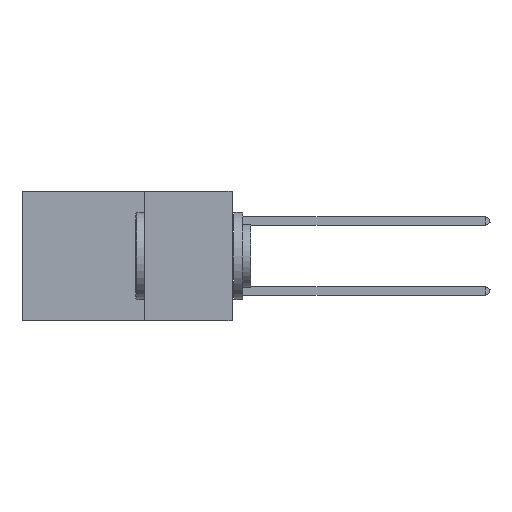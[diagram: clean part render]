
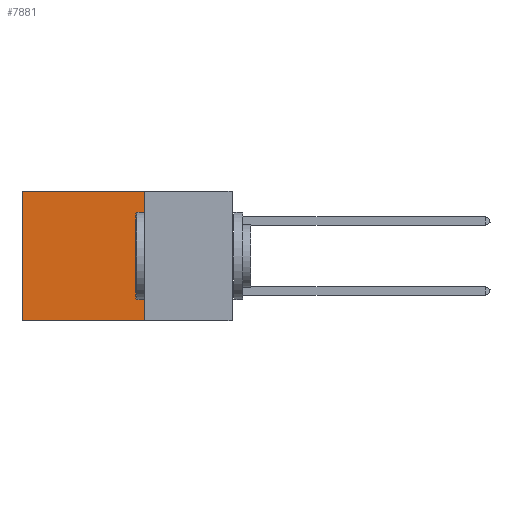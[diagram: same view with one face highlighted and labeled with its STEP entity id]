
A CAD part, left-side view. The second image highlights one B-rep face of the part: STEP entity #7881.
In plain terms, the highlighted planar face has unit normal (-1, 0, 0).
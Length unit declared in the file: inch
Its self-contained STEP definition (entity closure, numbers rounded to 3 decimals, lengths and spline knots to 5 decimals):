
#402 = VECTOR ( 'NONE', #1985, 39.37008 ) ;
#568 = LINE ( 'NONE', #24081, #28918 ) ;
#1506 = CARTESIAN_POINT ( 'NONE',  ( 0.2875, 0.6, 0. ) ) ;
#1723 = ORIENTED_EDGE ( 'NONE', *, *, #29041, .F. ) ;
#1985 = DIRECTION ( 'NONE',  ( 0., 0., -1. ) ) ;
#3082 = DIRECTION ( 'NONE',  ( 0., 1., 0. ) ) ;
#3548 = ORIENTED_EDGE ( 'NONE', *, *, #28963, .T. ) ;
#3559 = FACE_OUTER_BOUND ( 'NONE', #28014, .T. ) ;
#3706 = PLANE ( 'NONE',  #32171 ) ;
#4045 = CARTESIAN_POINT ( 'NONE',  ( 0.2875, 0.25, 0. ) ) ;
#6376 = CARTESIAN_POINT ( 'NONE',  ( 0.2875, 0.25, 0. ) ) ;
#7357 = VERTEX_POINT ( 'NONE', #14213 ) ;
#7756 = LINE ( 'NONE', #1506, #402 ) ;
#7881 = ADVANCED_FACE ( 'NONE', ( #3559 ), #3706, .F. ) ;
#9257 = CARTESIAN_POINT ( 'NONE',  ( 0.2875, 0.6, 0. ) ) ;
#11912 = DIRECTION ( 'NONE',  ( 1., 0., 0. ) ) ;
#13329 = LINE ( 'NONE', #15441, #30050 ) ;
#14213 = CARTESIAN_POINT ( 'NONE',  ( 0.2875, 0.25, -0.37 ) ) ;
#14477 = VERTEX_POINT ( 'NONE', #9257 ) ;
#15441 = CARTESIAN_POINT ( 'NONE',  ( 0.2875, 0.25, -0.37 ) ) ;
#18416 = DIRECTION ( 'NONE',  ( 0., 0., -1. ) ) ;
#18455 = DIRECTION ( 'NONE',  ( 0., 1., 0. ) ) ;
#20402 = CARTESIAN_POINT ( 'NONE',  ( 0.2875, 0.6, -0.37 ) ) ;
#20901 = VECTOR ( 'NONE', #3082, 39.37008 ) ;
#21437 = VERTEX_POINT ( 'NONE', #20402 ) ;
#22820 = DIRECTION ( 'NONE',  ( 0., 0., -1. ) ) ;
#23919 = LINE ( 'NONE', #4045, #20901 ) ;
#24081 = CARTESIAN_POINT ( 'NONE',  ( 0.2875, 0.25, 0. ) ) ;
#25894 = ORIENTED_EDGE ( 'NONE', *, *, #33479, .F. ) ;
#27419 = ORIENTED_EDGE ( 'NONE', *, *, #30746, .T. ) ;
#28014 = EDGE_LOOP ( 'NONE', ( #3548, #1723, #25894, #27419 ) ) ;
#28918 = VECTOR ( 'NONE', #18416, 39.37008 ) ;
#28963 = EDGE_CURVE ( 'NONE', #14477, #21437, #7756, .T. ) ;
#29041 = EDGE_CURVE ( 'NONE', #7357, #21437, #13329, .T. ) ;
#30050 = VECTOR ( 'NONE', #18455, 39.37008 ) ;
#30083 = CARTESIAN_POINT ( 'NONE',  ( 0.2875, 0.25, 0. ) ) ;
#30746 = EDGE_CURVE ( 'NONE', #33059, #14477, #23919, .T. ) ;
#32171 = AXIS2_PLACEMENT_3D ( 'NONE', #6376, #11912, #22820 ) ;
#33059 = VERTEX_POINT ( 'NONE', #30083 ) ;
#33479 = EDGE_CURVE ( 'NONE', #33059, #7357, #568, .T. ) ;
